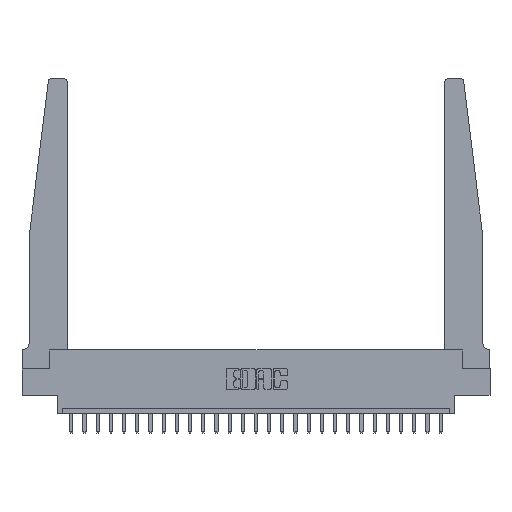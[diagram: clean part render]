
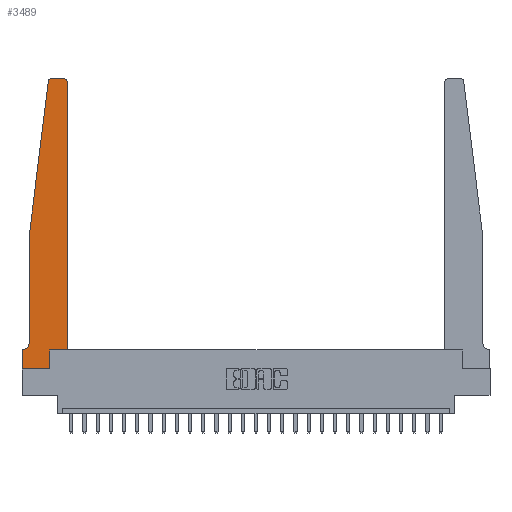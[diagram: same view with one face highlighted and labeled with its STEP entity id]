
A CAD part, top view. The second image highlights one B-rep face of the part: STEP entity #3489.
In plain terms, the highlighted planar face has unit normal (0, 0, 1).
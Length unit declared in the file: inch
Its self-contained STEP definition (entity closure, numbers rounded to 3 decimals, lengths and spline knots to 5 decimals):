
#89 = CARTESIAN_POINT ( 'NONE',  ( 0., 0.1875, 0.37 ) ) ;
#174 = EDGE_CURVE ( 'NONE', #9077, #12793, #18462, .T. ) ;
#303 = LINE ( 'NONE', #8571, #1793 ) ;
#340 = DIRECTION ( 'NONE',  ( -1., 0., 0. ) ) ;
#744 = DIRECTION ( 'NONE',  ( 1., 0., 0. ) ) ;
#1346 = CARTESIAN_POINT ( 'NONE',  ( 0.065, 1.25, 0.37 ) ) ;
#1521 = PLANE ( 'NONE',  #19000 ) ;
#1793 = VECTOR ( 'NONE', #10449, 39.37008 ) ;
#2295 = VERTEX_POINT ( 'NONE', #7457 ) ;
#3489 = ADVANCED_FACE ( 'NONE', ( #13867 ), #1521, .T. ) ;
#3527 = ORIENTED_EDGE ( 'NONE', *, *, #11453, .T. ) ;
#3773 = EDGE_CURVE ( 'NONE', #12331, #22679, #21851, .T. ) ;
#3927 = CARTESIAN_POINT ( 'NONE',  ( 0.015, 0.2375, 0.37 ) ) ;
#4371 = CARTESIAN_POINT ( 'NONE',  ( 0.065, 1.25, 0.37 ) ) ;
#4410 = DIRECTION ( 'NONE',  ( -1., 0., 0. ) ) ;
#4568 = CARTESIAN_POINT ( 'NONE',  ( 0.425, 2.72, 0.37 ) ) ;
#4772 = DIRECTION ( 'NONE',  ( 0., -1., 0. ) ) ;
#5078 = VERTEX_POINT ( 'NONE', #14738 ) ;
#5180 = CIRCLE ( 'NONE', #18211, 0.03 ) ;
#5239 = VECTOR ( 'NONE', #12686, 39.37008 ) ;
#5402 = VERTEX_POINT ( 'NONE', #89 ) ;
#5407 = CARTESIAN_POINT ( 'NONE',  ( 0.395, 2.72, 0.37 ) ) ;
#6004 = DIRECTION ( 'NONE',  ( 0., 0., -1. ) ) ;
#6531 = LINE ( 'NONE', #17364, #18532 ) ;
#6746 = VECTOR ( 'NONE', #4772, 39.37008 ) ;
#6835 = EDGE_CURVE ( 'NONE', #19937, #12331, #10342, .T. ) ;
#6851 = CARTESIAN_POINT ( 'NONE',  ( 0.425, 0.18, 0.37 ) ) ;
#7349 = CARTESIAN_POINT ( 'NONE',  ( 0.2605, 0.18, 0.37 ) ) ;
#7457 = CARTESIAN_POINT ( 'NONE',  ( 0.395, 2.75, 0.37 ) ) ;
#8066 = VECTOR ( 'NONE', #18582, 39.37008 ) ;
#8171 = ORIENTED_EDGE ( 'NONE', *, *, #10314, .T. ) ;
#8551 = ORIENTED_EDGE ( 'NONE', *, *, #3773, .T. ) ;
#8571 = CARTESIAN_POINT ( 'NONE',  ( 0., 0., 0.37 ) ) ;
#8776 = CARTESIAN_POINT ( 'NONE',  ( 0., 0., 0.37 ) ) ;
#9077 = VERTEX_POINT ( 'NONE', #11210 ) ;
#9126 = VECTOR ( 'NONE', #18342, 39.37008 ) ;
#9785 = CARTESIAN_POINT ( 'NONE',  ( 0.2605, 0.18, 0.37 ) ) ;
#10228 = CARTESIAN_POINT ( 'NONE',  ( 0.27653, 2.72, 0.37 ) ) ;
#10282 = VERTEX_POINT ( 'NONE', #17200 ) ;
#10302 = ORIENTED_EDGE ( 'NONE', *, *, #16223, .T. ) ;
#10314 = EDGE_CURVE ( 'NONE', #2295, #15615, #11959, .T. ) ;
#10342 = LINE ( 'NONE', #8776, #5239 ) ;
#10449 = DIRECTION ( 'NONE',  ( 0., -1., 0. ) ) ;
#11210 = CARTESIAN_POINT ( 'NONE',  ( 0.425, 0.18, 0.37 ) ) ;
#11453 = EDGE_CURVE ( 'NONE', #15615, #5078, #5180, .T. ) ;
#11531 = EDGE_CURVE ( 'NONE', #5078, #23832, #20164, .T. ) ;
#11750 = CARTESIAN_POINT ( 'NONE',  ( 0.015, 0.1875, 0.37 ) ) ;
#11802 = ORIENTED_EDGE ( 'NONE', *, *, #23639, .T. ) ;
#11959 = LINE ( 'NONE', #13622, #17069 ) ;
#12016 = AXIS2_PLACEMENT_3D ( 'NONE', #5407, #12884, #12359 ) ;
#12331 = VERTEX_POINT ( 'NONE', #15090 ) ;
#12359 = DIRECTION ( 'NONE',  ( 1., 0., 0. ) ) ;
#12522 = CIRCLE ( 'NONE', #12016, 0.03 ) ;
#12686 = DIRECTION ( 'NONE',  ( 1., 0., 0. ) ) ;
#12793 = VERTEX_POINT ( 'NONE', #4568 ) ;
#12884 = DIRECTION ( 'NONE',  ( 0., 0., 1. ) ) ;
#13290 = DIRECTION ( 'NONE',  ( 0., 0., 1. ) ) ;
#13622 = CARTESIAN_POINT ( 'NONE',  ( 0.25, 2.75, 0.37 ) ) ;
#13665 = ORIENTED_EDGE ( 'NONE', *, *, #14492, .T. ) ;
#13867 = FACE_OUTER_BOUND ( 'NONE', #16637, .T. ) ;
#13945 = DIRECTION ( 'NONE',  ( 0., 0., 1. ) ) ;
#14492 = EDGE_CURVE ( 'NONE', #22679, #9077, #6531, .T. ) ;
#14738 = CARTESIAN_POINT ( 'NONE',  ( 0.24675, 2.72367, 0.37 ) ) ;
#14911 = CIRCLE ( 'NONE', #18337, 0.05 ) ;
#15090 = CARTESIAN_POINT ( 'NONE',  ( 0.2605, 0., 0.37 ) ) ;
#15161 = LINE ( 'NONE', #15902, #24053 ) ;
#15505 = EDGE_CURVE ( 'NONE', #12793, #2295, #12522, .T. ) ;
#15615 = VERTEX_POINT ( 'NONE', #19208 ) ;
#15826 = ORIENTED_EDGE ( 'NONE', *, *, #19545, .T. ) ;
#15897 = VERTEX_POINT ( 'NONE', #11750 ) ;
#15902 = CARTESIAN_POINT ( 'NONE',  ( 0.065, 0.1875, 0.37 ) ) ;
#16223 = EDGE_CURVE ( 'NONE', #23832, #10282, #24103, .T. ) ;
#16637 = EDGE_LOOP ( 'NONE', ( #8171, #3527, #20179, #10302, #23567, #11802, #15826, #23450, #8551, #13665, #22576, #24611 ) ) ;
#17048 = CARTESIAN_POINT ( 'NONE',  ( 0., 0.1875, 0.37 ) ) ;
#17069 = VECTOR ( 'NONE', #340, 39.37008 ) ;
#17115 = DIRECTION ( 'NONE',  ( 1., 0., 0. ) ) ;
#17200 = CARTESIAN_POINT ( 'NONE',  ( 0.065, 0.2375, 0.37 ) ) ;
#17364 = CARTESIAN_POINT ( 'NONE',  ( 0.425, 0.18, 0.37 ) ) ;
#17804 = CARTESIAN_POINT ( 'NONE',  ( 0., 0., 0.37 ) ) ;
#18211 = AXIS2_PLACEMENT_3D ( 'NONE', #10228, #13945, #744 ) ;
#18337 = AXIS2_PLACEMENT_3D ( 'NONE', #3927, #6004, #19400 ) ;
#18342 = DIRECTION ( 'NONE',  ( 0., 1., 0. ) ) ;
#18462 = LINE ( 'NONE', #6851, #9126 ) ;
#18532 = VECTOR ( 'NONE', #17115, 39.37008 ) ;
#18582 = DIRECTION ( 'NONE',  ( 0., 1., 0. ) ) ;
#19000 = AXIS2_PLACEMENT_3D ( 'NONE', #17048, #13290, #19173 ) ;
#19173 = DIRECTION ( 'NONE',  ( 1., 0., 0. ) ) ;
#19208 = CARTESIAN_POINT ( 'NONE',  ( 0.27653, 2.75, 0.37 ) ) ;
#19400 = DIRECTION ( 'NONE',  ( -1., 0., 0. ) ) ;
#19545 = EDGE_CURVE ( 'NONE', #5402, #19937, #303, .T. ) ;
#19820 = CARTESIAN_POINT ( 'NONE',  ( 0.065, 1.25, 0.37 ) ) ;
#19937 = VERTEX_POINT ( 'NONE', #17804 ) ;
#20164 = LINE ( 'NONE', #4371, #22817 ) ;
#20179 = ORIENTED_EDGE ( 'NONE', *, *, #11531, .T. ) ;
#21728 = DIRECTION ( 'NONE',  ( -0.122, -0.992, 0. ) ) ;
#21851 = LINE ( 'NONE', #7349, #8066 ) ;
#22186 = EDGE_CURVE ( 'NONE', #10282, #15897, #14911, .T. ) ;
#22576 = ORIENTED_EDGE ( 'NONE', *, *, #174, .T. ) ;
#22679 = VERTEX_POINT ( 'NONE', #9785 ) ;
#22817 = VECTOR ( 'NONE', #21728, 39.37008 ) ;
#23450 = ORIENTED_EDGE ( 'NONE', *, *, #6835, .T. ) ;
#23567 = ORIENTED_EDGE ( 'NONE', *, *, #22186, .T. ) ;
#23639 = EDGE_CURVE ( 'NONE', #15897, #5402, #15161, .T. ) ;
#23832 = VERTEX_POINT ( 'NONE', #1346 ) ;
#24053 = VECTOR ( 'NONE', #4410, 39.37008 ) ;
#24103 = LINE ( 'NONE', #19820, #6746 ) ;
#24611 = ORIENTED_EDGE ( 'NONE', *, *, #15505, .T. ) ;
